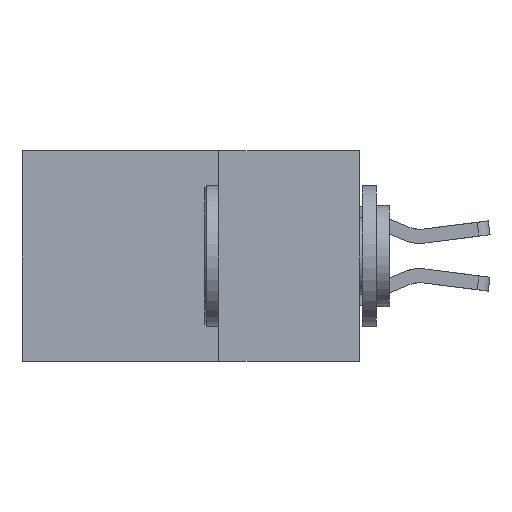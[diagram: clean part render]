
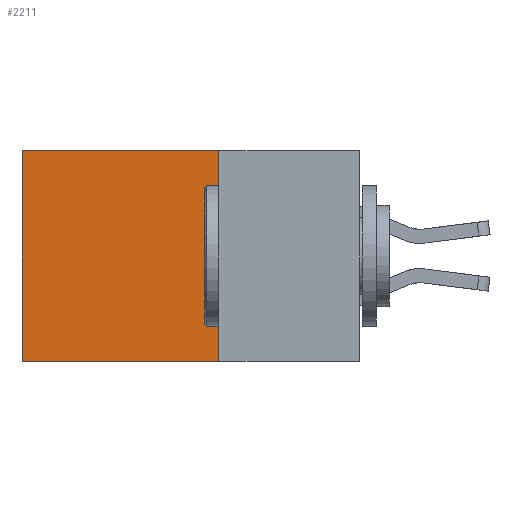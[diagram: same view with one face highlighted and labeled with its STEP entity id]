
A CAD part, left-side view. The second image highlights one B-rep face of the part: STEP entity #2211.
In plain terms, the highlighted planar face has unit normal (-1, 0, 0).
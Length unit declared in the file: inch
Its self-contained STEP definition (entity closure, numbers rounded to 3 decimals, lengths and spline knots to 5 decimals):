
#32 = LINE ( 'NONE', #8462, #2336 ) ;
#156 = DIRECTION ( 'NONE',  ( 0., 0., -1. ) ) ;
#1083 = CARTESIAN_POINT ( 'NONE',  ( 0.2875, 0.6, -0.375 ) ) ;
#1495 = EDGE_CURVE ( 'NONE', #6272, #5759, #2479, .T. ) ;
#1610 = ORIENTED_EDGE ( 'NONE', *, *, #4574, .F. ) ;
#2211 = ADVANCED_FACE ( 'NONE', ( #6062 ), #2442, .F. ) ;
#2336 = VECTOR ( 'NONE', #4206, 39.37008 ) ;
#2424 = CARTESIAN_POINT ( 'NONE',  ( 0.2875, 0.25, 0. ) ) ;
#2433 = EDGE_CURVE ( 'NONE', #6272, #7970, #9152, .T. ) ;
#2442 = PLANE ( 'NONE',  #6757 ) ;
#2479 = LINE ( 'NONE', #2424, #6176 ) ;
#3110 = ORIENTED_EDGE ( 'NONE', *, *, #2433, .F. ) ;
#3184 = DIRECTION ( 'NONE',  ( 0., 1., 0. ) ) ;
#3903 = VERTEX_POINT ( 'NONE', #1083 ) ;
#4013 = EDGE_CURVE ( 'NONE', #5759, #3903, #32, .T. ) ;
#4206 = DIRECTION ( 'NONE',  ( 0., 0., -1. ) ) ;
#4361 = DIRECTION ( 'NONE',  ( 0., 1., 0. ) ) ;
#4503 = LINE ( 'NONE', #9434, #9113 ) ;
#4548 = DIRECTION ( 'NONE',  ( 1., 0., 0. ) ) ;
#4574 = EDGE_CURVE ( 'NONE', #7970, #3903, #4503, .T. ) ;
#5250 = VECTOR ( 'NONE', #5599, 39.37008 ) ;
#5599 = DIRECTION ( 'NONE',  ( 0., 0., -1. ) ) ;
#5682 = CARTESIAN_POINT ( 'NONE',  ( 0.2875, 0.25, -0.375 ) ) ;
#5759 = VERTEX_POINT ( 'NONE', #7843 ) ;
#6062 = FACE_OUTER_BOUND ( 'NONE', #8836, .T. ) ;
#6176 = VECTOR ( 'NONE', #3184, 39.37008 ) ;
#6272 = VERTEX_POINT ( 'NONE', #7177 ) ;
#6343 = ORIENTED_EDGE ( 'NONE', *, *, #4013, .T. ) ;
#6757 = AXIS2_PLACEMENT_3D ( 'NONE', #7491, #4548, #156 ) ;
#7177 = CARTESIAN_POINT ( 'NONE',  ( 0.2875, 0.25, 0. ) ) ;
#7454 = ORIENTED_EDGE ( 'NONE', *, *, #1495, .T. ) ;
#7491 = CARTESIAN_POINT ( 'NONE',  ( 0.2875, 0.25, -0.375 ) ) ;
#7836 = CARTESIAN_POINT ( 'NONE',  ( 0.2875, 0.25, -0.375 ) ) ;
#7843 = CARTESIAN_POINT ( 'NONE',  ( 0.2875, 0.6, 0. ) ) ;
#7970 = VERTEX_POINT ( 'NONE', #5682 ) ;
#8462 = CARTESIAN_POINT ( 'NONE',  ( 0.2875, 0.6, -0.375 ) ) ;
#8836 = EDGE_LOOP ( 'NONE', ( #6343, #1610, #3110, #7454 ) ) ;
#9113 = VECTOR ( 'NONE', #4361, 39.37008 ) ;
#9152 = LINE ( 'NONE', #7836, #5250 ) ;
#9434 = CARTESIAN_POINT ( 'NONE',  ( 0.2875, 0.25, -0.375 ) ) ;
